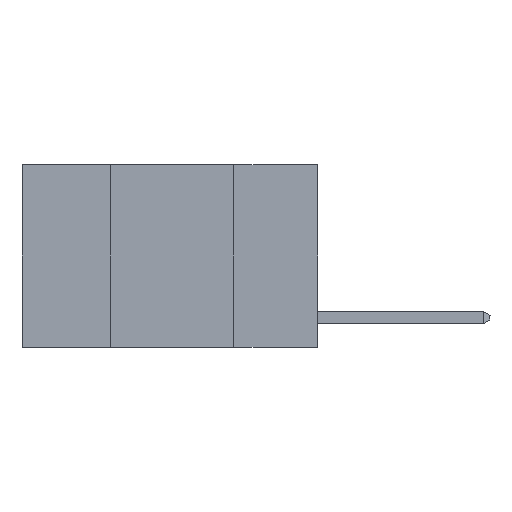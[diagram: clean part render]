
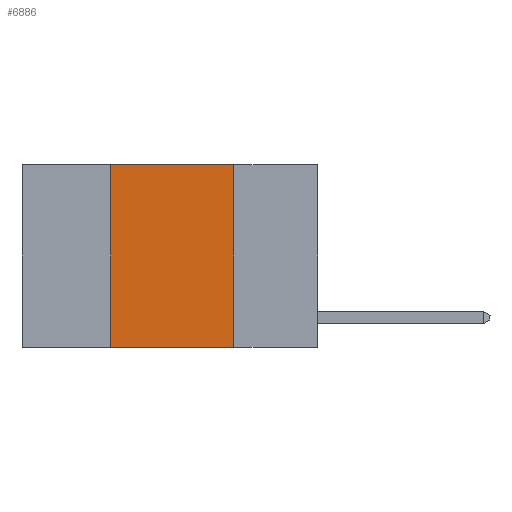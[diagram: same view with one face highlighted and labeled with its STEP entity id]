
A CAD part, left-side view. The second image highlights one B-rep face of the part: STEP entity #6886.
In plain terms, the highlighted planar face has unit normal (-1, 0, 0).
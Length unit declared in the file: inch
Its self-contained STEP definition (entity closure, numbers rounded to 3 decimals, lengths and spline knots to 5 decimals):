
#5 = VERTEX_POINT ( 'NONE', #3902 ) ;
#70 = DIRECTION ( 'NONE',  ( 0., 0., -1. ) ) ;
#355 = ORIENTED_EDGE ( 'NONE', *, *, #4256, .F. ) ;
#1108 = LINE ( 'NONE', #6649, #10553 ) ;
#1826 = VECTOR ( 'NONE', #70, 39.37008 ) ;
#1885 = DIRECTION ( 'NONE',  ( 0., -1., 0. ) ) ;
#2959 = FACE_OUTER_BOUND ( 'NONE', #5950, .T. ) ;
#3230 = ORIENTED_EDGE ( 'NONE', *, *, #9402, .F. ) ;
#3902 = CARTESIAN_POINT ( 'NONE',  ( 0., 0.17, 0. ) ) ;
#3952 = DIRECTION ( 'NONE',  ( 0., 0., -1. ) ) ;
#4152 = AXIS2_PLACEMENT_3D ( 'NONE', #7562, #9349, #3952 ) ;
#4256 = EDGE_CURVE ( 'NONE', #5, #7501, #9409, .T. ) ;
#4442 = LINE ( 'NONE', #10095, #9495 ) ;
#4862 = PLANE ( 'NONE',  #4152 ) ;
#5336 = ORIENTED_EDGE ( 'NONE', *, *, #6768, .T. ) ;
#5670 = VECTOR ( 'NONE', #11658, 39.37008 ) ;
#5950 = EDGE_LOOP ( 'NONE', ( #355, #3230, #8181, #5336 ) ) ;
#6649 = CARTESIAN_POINT ( 'NONE',  ( 0., 0.6, 0. ) ) ;
#6706 = CARTESIAN_POINT ( 'NONE',  ( 0., 0.17, 0. ) ) ;
#6768 = EDGE_CURVE ( 'NONE', #6843, #7501, #4442, .T. ) ;
#6843 = VERTEX_POINT ( 'NONE', #7531 ) ;
#6886 = ADVANCED_FACE ( 'NONE', ( #2959 ), #4862, .F. ) ;
#7501 = VERTEX_POINT ( 'NONE', #11848 ) ;
#7531 = CARTESIAN_POINT ( 'NONE',  ( 0., 0.42, -0.37 ) ) ;
#7562 = CARTESIAN_POINT ( 'NONE',  ( 0., 0.6, 0. ) ) ;
#8028 = LINE ( 'NONE', #9936, #5670 ) ;
#8181 = ORIENTED_EDGE ( 'NONE', *, *, #10980, .F. ) ;
#9349 = DIRECTION ( 'NONE',  ( 1., 0., 0. ) ) ;
#9402 = EDGE_CURVE ( 'NONE', #9639, #5, #1108, .T. ) ;
#9409 = LINE ( 'NONE', #6706, #1826 ) ;
#9495 = VECTOR ( 'NONE', #1885, 39.37008 ) ;
#9639 = VERTEX_POINT ( 'NONE', #11332 ) ;
#9936 = CARTESIAN_POINT ( 'NONE',  ( 0., 0.42, 0. ) ) ;
#10095 = CARTESIAN_POINT ( 'NONE',  ( 0., 0.6, -0.37 ) ) ;
#10187 = DIRECTION ( 'NONE',  ( 0., -1., 0. ) ) ;
#10553 = VECTOR ( 'NONE', #10187, 39.37008 ) ;
#10980 = EDGE_CURVE ( 'NONE', #6843, #9639, #8028, .T. ) ;
#11332 = CARTESIAN_POINT ( 'NONE',  ( 0., 0.42, 0. ) ) ;
#11658 = DIRECTION ( 'NONE',  ( 0., 0., 1. ) ) ;
#11848 = CARTESIAN_POINT ( 'NONE',  ( 0., 0.17, -0.37 ) ) ;
